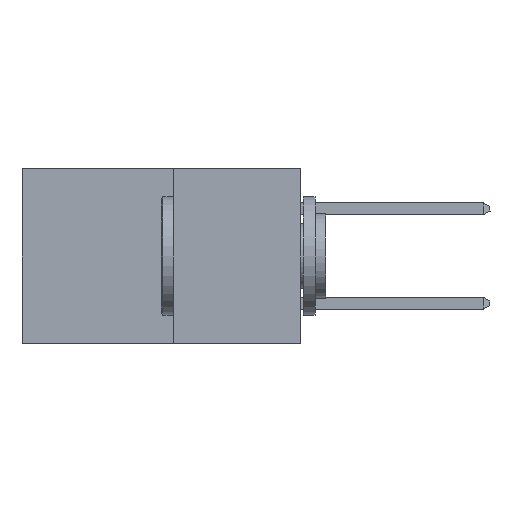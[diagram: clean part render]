
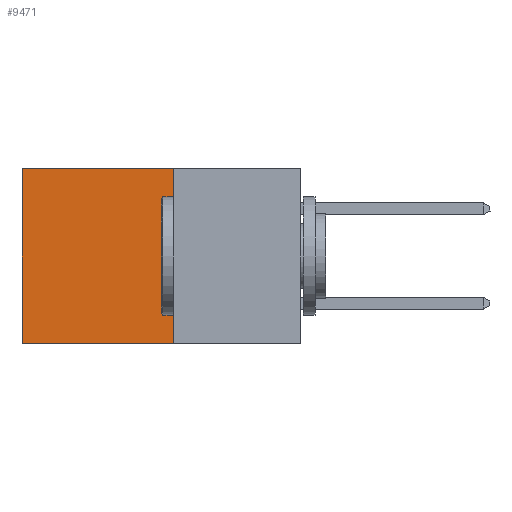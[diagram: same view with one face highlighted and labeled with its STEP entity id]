
A CAD part, left-side view. The second image highlights one B-rep face of the part: STEP entity #9471.
In plain terms, the highlighted planar face has unit normal (-1, 0, 0).
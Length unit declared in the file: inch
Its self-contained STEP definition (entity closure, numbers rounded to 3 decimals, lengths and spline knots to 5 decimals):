
#750 = DIRECTION ( 'NONE',  ( 0., 0., -1. ) ) ;
#1993 = CARTESIAN_POINT ( 'NONE',  ( 0.277, 0.59, 0. ) ) ;
#2064 = EDGE_CURVE ( 'NONE', #19892, #22329, #21642, .T. ) ;
#2120 = VECTOR ( 'NONE', #27858, 39.37008 ) ;
#2455 = FACE_OUTER_BOUND ( 'NONE', #23819, .T. ) ;
#3011 = LINE ( 'NONE', #4969, #14921 ) ;
#4810 = CARTESIAN_POINT ( 'NONE',  ( 0.277, 0.27, -0.37 ) ) ;
#4892 = DIRECTION ( 'NONE',  ( 0., 0., -1. ) ) ;
#4969 = CARTESIAN_POINT ( 'NONE',  ( 0.277, 0.59, -0.37 ) ) ;
#5047 = EDGE_CURVE ( 'NONE', #22329, #21676, #3011, .T. ) ;
#5607 = CARTESIAN_POINT ( 'NONE',  ( 0.277, 0.27, -0.37 ) ) ;
#6224 = ORIENTED_EDGE ( 'NONE', *, *, #28923, .F. ) ;
#7276 = CARTESIAN_POINT ( 'NONE',  ( 0.277, 0.59, -0.37 ) ) ;
#8429 = CARTESIAN_POINT ( 'NONE',  ( 0.277, 0.27, -0.37 ) ) ;
#9471 = ADVANCED_FACE ( 'NONE', ( #2455 ), #11869, .F. ) ;
#11802 = DIRECTION ( 'NONE',  ( 0., 0., -1. ) ) ;
#11831 = DIRECTION ( 'NONE',  ( 1., 0., 0. ) ) ;
#11869 = PLANE ( 'NONE',  #26034 ) ;
#12502 = CARTESIAN_POINT ( 'NONE',  ( 0.277, 0.27, -0.37 ) ) ;
#12835 = VERTEX_POINT ( 'NONE', #5607 ) ;
#14921 = VECTOR ( 'NONE', #4892, 39.37008 ) ;
#16538 = CARTESIAN_POINT ( 'NONE',  ( 0.277, 0.27, 0. ) ) ;
#16971 = EDGE_CURVE ( 'NONE', #19892, #12835, #31992, .T. ) ;
#18040 = VECTOR ( 'NONE', #25081, 39.37008 ) ;
#19456 = VECTOR ( 'NONE', #750, 39.37008 ) ;
#19651 = LINE ( 'NONE', #4810, #18040 ) ;
#19892 = VERTEX_POINT ( 'NONE', #23169 ) ;
#21642 = LINE ( 'NONE', #16538, #2120 ) ;
#21676 = VERTEX_POINT ( 'NONE', #7276 ) ;
#22329 = VERTEX_POINT ( 'NONE', #1993 ) ;
#23169 = CARTESIAN_POINT ( 'NONE',  ( 0.277, 0.27, 0. ) ) ;
#23819 = EDGE_LOOP ( 'NONE', ( #29013, #6224, #31616, #28852 ) ) ;
#25081 = DIRECTION ( 'NONE',  ( 0., 1., 0. ) ) ;
#26034 = AXIS2_PLACEMENT_3D ( 'NONE', #12502, #11831, #11802 ) ;
#27858 = DIRECTION ( 'NONE',  ( 0., 1., 0. ) ) ;
#28852 = ORIENTED_EDGE ( 'NONE', *, *, #2064, .T. ) ;
#28923 = EDGE_CURVE ( 'NONE', #12835, #21676, #19651, .T. ) ;
#29013 = ORIENTED_EDGE ( 'NONE', *, *, #5047, .T. ) ;
#31616 = ORIENTED_EDGE ( 'NONE', *, *, #16971, .F. ) ;
#31992 = LINE ( 'NONE', #8429, #19456 ) ;
